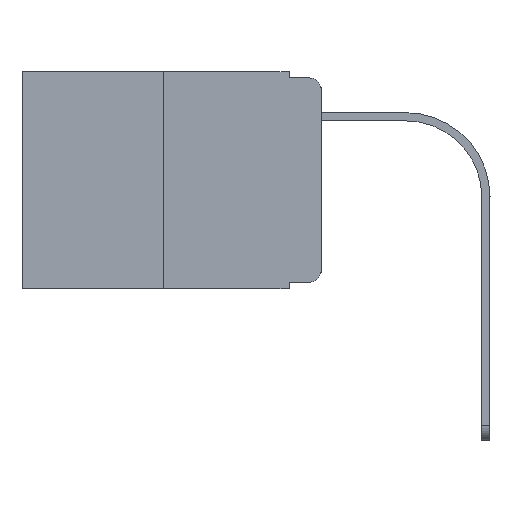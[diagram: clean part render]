
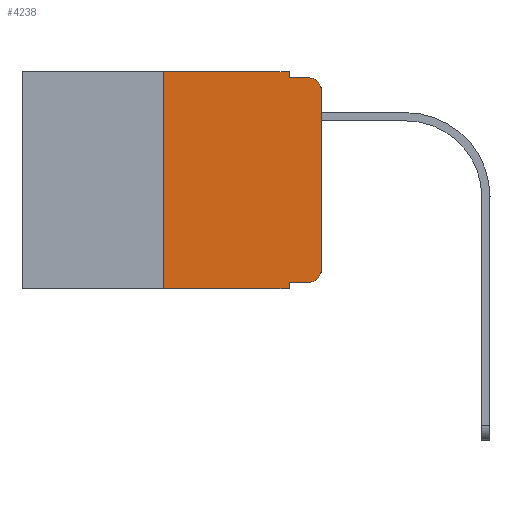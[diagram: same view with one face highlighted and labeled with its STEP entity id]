
A CAD part, left-side view. The second image highlights one B-rep face of the part: STEP entity #4238.
In plain terms, the highlighted planar face has unit normal (-1, 0, 0).
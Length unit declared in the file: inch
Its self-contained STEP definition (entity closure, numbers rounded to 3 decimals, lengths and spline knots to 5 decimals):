
#92 = VECTOR ( 'NONE', #8888, 39.37008 ) ;
#179 = LINE ( 'NONE', #6191, #9481 ) ;
#292 = ORIENTED_EDGE ( 'NONE', *, *, #6018, .F. ) ;
#318 = CARTESIAN_POINT ( 'NONE',  ( 0., 0.051, -0.343 ) ) ;
#341 = LINE ( 'NONE', #1026, #3508 ) ;
#358 = DIRECTION ( 'NONE',  ( 0., 0., -1. ) ) ;
#398 = EDGE_CURVE ( 'NONE', #7124, #9279, #8966, .T. ) ;
#602 = ORIENTED_EDGE ( 'NONE', *, *, #3867, .F. ) ;
#619 = DIRECTION ( 'NONE',  ( 1., 0., 0. ) ) ;
#719 = EDGE_CURVE ( 'NONE', #7393, #9167, #341, .T. ) ;
#747 = CARTESIAN_POINT ( 'NONE',  ( 0., 0.473, 0. ) ) ;
#792 = DIRECTION ( 'NONE',  ( 0., 0., -1. ) ) ;
#793 = DIRECTION ( 'NONE',  ( 0., 0., 1. ) ) ;
#820 = ORIENTED_EDGE ( 'NONE', *, *, #398, .T. ) ;
#920 = ORIENTED_EDGE ( 'NONE', *, *, #6339, .F. ) ;
#990 = CARTESIAN_POINT ( 'NONE',  ( 0., 0.02, -0.03 ) ) ;
#1026 = CARTESIAN_POINT ( 'NONE',  ( 0., 0.051, 0. ) ) ;
#1098 = CARTESIAN_POINT ( 'NONE',  ( 0., 0., -0.03 ) ) ;
#1313 = CARTESIAN_POINT ( 'NONE',  ( 0., 0.051, -0.01 ) ) ;
#1346 = EDGE_CURVE ( 'NONE', #7904, #1607, #1792, .T. ) ;
#1607 = VERTEX_POINT ( 'NONE', #6720 ) ;
#1694 = ORIENTED_EDGE ( 'NONE', *, *, #1842, .T. ) ;
#1699 = CARTESIAN_POINT ( 'NONE',  ( 0., 0.051, 0. ) ) ;
#1743 = ORIENTED_EDGE ( 'NONE', *, *, #6692, .F. ) ;
#1792 = CIRCLE ( 'NONE', #9157, 0.02 ) ;
#1842 = EDGE_CURVE ( 'NONE', #7393, #7904, #7837, .T. ) ;
#1945 = CARTESIAN_POINT ( 'NONE',  ( 0., 0., 0. ) ) ;
#2017 = VECTOR ( 'NONE', #8525, 39.37008 ) ;
#2217 = CARTESIAN_POINT ( 'NONE',  ( 0., 0.473, 0. ) ) ;
#2510 = CARTESIAN_POINT ( 'NONE',  ( 0., 0.051, -0.333 ) ) ;
#2688 = LINE ( 'NONE', #1945, #8723 ) ;
#2798 = DIRECTION ( 'NONE',  ( 0., 0., 1. ) ) ;
#3153 = CARTESIAN_POINT ( 'NONE',  ( 0., 0.25, 0. ) ) ;
#3214 = VERTEX_POINT ( 'NONE', #3153 ) ;
#3476 = CARTESIAN_POINT ( 'NONE',  ( 0., 0.02, -0.333 ) ) ;
#3508 = VECTOR ( 'NONE', #6910, 39.37008 ) ;
#3666 = FACE_OUTER_BOUND ( 'NONE', #7674, .T. ) ;
#3708 = EDGE_CURVE ( 'NONE', #1607, #7124, #2688, .T. ) ;
#3758 = DIRECTION ( 'NONE',  ( 0., -1., 0. ) ) ;
#3867 = EDGE_CURVE ( 'NONE', #8005, #7832, #6843, .T. ) ;
#4012 = DIRECTION ( 'NONE',  ( 0., 0., -1. ) ) ;
#4114 = CARTESIAN_POINT ( 'NONE',  ( 0., 0.02, -0.313 ) ) ;
#4238 = ADVANCED_FACE ( 'NONE', ( #3666 ), #5929, .F. ) ;
#4353 = CARTESIAN_POINT ( 'NONE',  ( 0., 0.473, -0.343 ) ) ;
#4749 = CARTESIAN_POINT ( 'NONE',  ( 0., 0.25, -0.343 ) ) ;
#5043 = VERTEX_POINT ( 'NONE', #4749 ) ;
#5072 = AXIS2_PLACEMENT_3D ( 'NONE', #990, #7069, #4012 ) ;
#5929 = PLANE ( 'NONE',  #8881 ) ;
#6018 = EDGE_CURVE ( 'NONE', #5043, #3214, #6023, .T. ) ;
#6023 = LINE ( 'NONE', #6124, #9343 ) ;
#6073 = VECTOR ( 'NONE', #6276, 39.37008 ) ;
#6124 = CARTESIAN_POINT ( 'NONE',  ( 0., 0.25, 0. ) ) ;
#6191 = CARTESIAN_POINT ( 'NONE',  ( 0., 0.051, -0.01 ) ) ;
#6276 = DIRECTION ( 'NONE',  ( 0., 0., -1. ) ) ;
#6339 = EDGE_CURVE ( 'NONE', #3214, #8005, #8198, .T. ) ;
#6692 = EDGE_CURVE ( 'NONE', #7832, #9279, #179, .T. ) ;
#6720 = CARTESIAN_POINT ( 'NONE',  ( 0., 0., -0.313 ) ) ;
#6747 = CARTESIAN_POINT ( 'NONE',  ( 0., 0.051, 0. ) ) ;
#6843 = LINE ( 'NONE', #1699, #6073 ) ;
#6910 = DIRECTION ( 'NONE',  ( 0., 0., -1. ) ) ;
#7069 = DIRECTION ( 'NONE',  ( -1., 0., 0. ) ) ;
#7124 = VERTEX_POINT ( 'NONE', #1098 ) ;
#7393 = VERTEX_POINT ( 'NONE', #2510 ) ;
#7474 = CARTESIAN_POINT ( 'NONE',  ( 0., 0.02, -0.01 ) ) ;
#7604 = ORIENTED_EDGE ( 'NONE', *, *, #1346, .T. ) ;
#7674 = EDGE_LOOP ( 'NONE', ( #8875, #820, #1743, #602, #920, #292, #8439, #8722, #1694, #7604 ) ) ;
#7832 = VERTEX_POINT ( 'NONE', #1313 ) ;
#7837 = LINE ( 'NONE', #8669, #2017 ) ;
#7904 = VERTEX_POINT ( 'NONE', #3476 ) ;
#7958 = LINE ( 'NONE', #4353, #92 ) ;
#8005 = VERTEX_POINT ( 'NONE', #6747 ) ;
#8198 = LINE ( 'NONE', #747, #9350 ) ;
#8439 = ORIENTED_EDGE ( 'NONE', *, *, #8774, .T. ) ;
#8525 = DIRECTION ( 'NONE',  ( 0., -1., 0. ) ) ;
#8601 = DIRECTION ( 'NONE',  ( -1., 0., 0. ) ) ;
#8669 = CARTESIAN_POINT ( 'NONE',  ( 0., 0.051, -0.333 ) ) ;
#8722 = ORIENTED_EDGE ( 'NONE', *, *, #719, .F. ) ;
#8723 = VECTOR ( 'NONE', #2798, 39.37008 ) ;
#8774 = EDGE_CURVE ( 'NONE', #5043, #9167, #7958, .T. ) ;
#8875 = ORIENTED_EDGE ( 'NONE', *, *, #3708, .T. ) ;
#8881 = AXIS2_PLACEMENT_3D ( 'NONE', #2217, #619, #792 ) ;
#8888 = DIRECTION ( 'NONE',  ( 0., -1., 0. ) ) ;
#8966 = CIRCLE ( 'NONE', #5072, 0.02 ) ;
#9157 = AXIS2_PLACEMENT_3D ( 'NONE', #4114, #8601, #358 ) ;
#9161 = DIRECTION ( 'NONE',  ( 0., -1., 0. ) ) ;
#9167 = VERTEX_POINT ( 'NONE', #318 ) ;
#9279 = VERTEX_POINT ( 'NONE', #7474 ) ;
#9343 = VECTOR ( 'NONE', #793, 39.37008 ) ;
#9350 = VECTOR ( 'NONE', #3758, 39.37008 ) ;
#9481 = VECTOR ( 'NONE', #9161, 39.37008 ) ;
